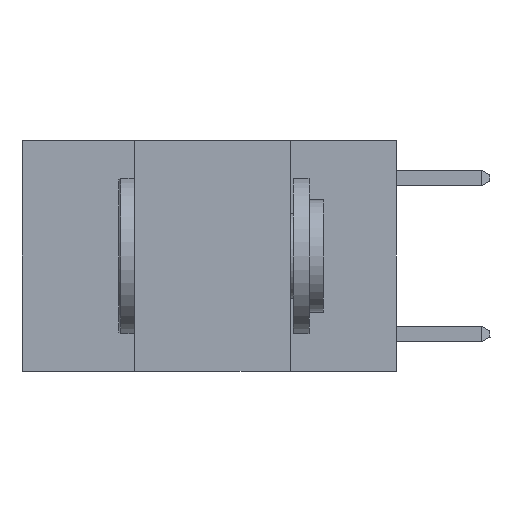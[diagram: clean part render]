
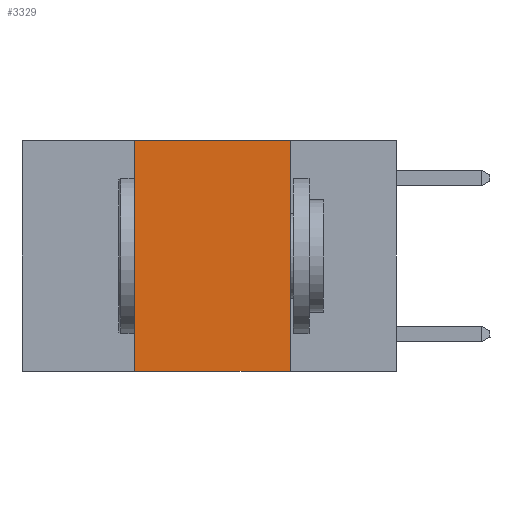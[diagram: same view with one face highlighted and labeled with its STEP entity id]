
A CAD part, left-side view. The second image highlights one B-rep face of the part: STEP entity #3329.
In plain terms, the highlighted planar face has unit normal (-1, 0, 0).
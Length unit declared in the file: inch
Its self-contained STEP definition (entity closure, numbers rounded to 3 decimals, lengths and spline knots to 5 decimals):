
#88 = LINE ( 'NONE', #6079, #7790 ) ;
#185 = PLANE ( 'NONE',  #6586 ) ;
#491 = LINE ( 'NONE', #13381, #3057 ) ;
#1177 = DIRECTION ( 'NONE',  ( 0., 0., 1. ) ) ;
#1772 = CARTESIAN_POINT ( 'NONE',  ( 0., 0.17, 0. ) ) ;
#1997 = EDGE_CURVE ( 'NONE', #4085, #7573, #88, .T. ) ;
#3057 = VECTOR ( 'NONE', #4025, 39.37008 ) ;
#3329 = ADVANCED_FACE ( 'NONE', ( #8487 ), #185, .F. ) ;
#4025 = DIRECTION ( 'NONE',  ( 0., -1., 0. ) ) ;
#4085 = VERTEX_POINT ( 'NONE', #13256 ) ;
#4325 = ORIENTED_EDGE ( 'NONE', *, *, #1997, .F. ) ;
#4460 = ORIENTED_EDGE ( 'NONE', *, *, #12226, .T. ) ;
#4759 = CARTESIAN_POINT ( 'NONE',  ( 0., 0.17, -0.37 ) ) ;
#4871 = CARTESIAN_POINT ( 'NONE',  ( 0., 0.6, 0. ) ) ;
#4905 = LINE ( 'NONE', #11878, #9330 ) ;
#5573 = ORIENTED_EDGE ( 'NONE', *, *, #13244, .F. ) ;
#6005 = EDGE_CURVE ( 'NONE', #7573, #14708, #4905, .T. ) ;
#6022 = VECTOR ( 'NONE', #6459, 39.37008 ) ;
#6079 = CARTESIAN_POINT ( 'NONE',  ( 0., 0.42, 0. ) ) ;
#6459 = DIRECTION ( 'NONE',  ( 0., 0., -1. ) ) ;
#6586 = AXIS2_PLACEMENT_3D ( 'NONE', #4871, #9562, #13081 ) ;
#7573 = VERTEX_POINT ( 'NONE', #13347 ) ;
#7790 = VECTOR ( 'NONE', #1177, 39.37008 ) ;
#7985 = CARTESIAN_POINT ( 'NONE',  ( 0., 0.17, 0. ) ) ;
#8487 = FACE_OUTER_BOUND ( 'NONE', #12800, .T. ) ;
#9330 = VECTOR ( 'NONE', #10427, 39.37008 ) ;
#9562 = DIRECTION ( 'NONE',  ( 1., 0., 0. ) ) ;
#10319 = ORIENTED_EDGE ( 'NONE', *, *, #6005, .F. ) ;
#10427 = DIRECTION ( 'NONE',  ( 0., -1., 0. ) ) ;
#11049 = LINE ( 'NONE', #1772, #6022 ) ;
#11878 = CARTESIAN_POINT ( 'NONE',  ( 0., 0.6, 0. ) ) ;
#12226 = EDGE_CURVE ( 'NONE', #4085, #13010, #491, .T. ) ;
#12800 = EDGE_LOOP ( 'NONE', ( #5573, #10319, #4325, #4460 ) ) ;
#13010 = VERTEX_POINT ( 'NONE', #4759 ) ;
#13081 = DIRECTION ( 'NONE',  ( 0., 0., -1. ) ) ;
#13244 = EDGE_CURVE ( 'NONE', #14708, #13010, #11049, .T. ) ;
#13256 = CARTESIAN_POINT ( 'NONE',  ( 0., 0.42, -0.37 ) ) ;
#13347 = CARTESIAN_POINT ( 'NONE',  ( 0., 0.42, 0. ) ) ;
#13381 = CARTESIAN_POINT ( 'NONE',  ( 0., 0.6, -0.37 ) ) ;
#14708 = VERTEX_POINT ( 'NONE', #7985 ) ;
